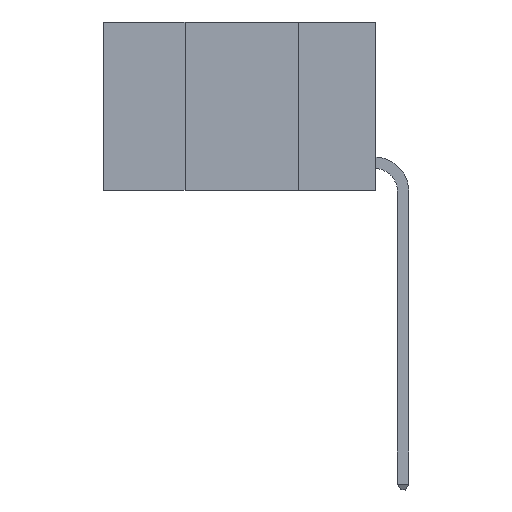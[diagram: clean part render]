
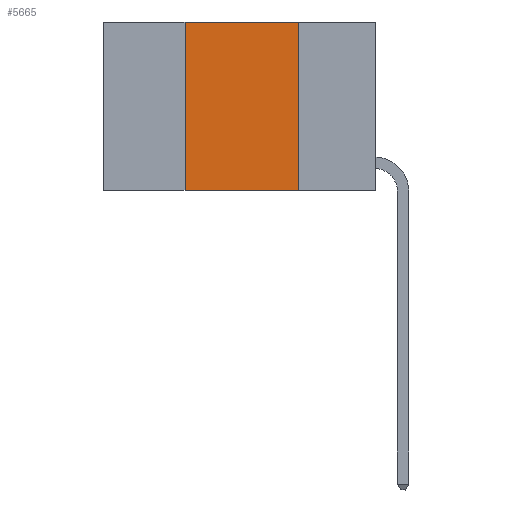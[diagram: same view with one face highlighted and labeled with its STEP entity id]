
A CAD part, left-side view. The second image highlights one B-rep face of the part: STEP entity #5665.
In plain terms, the highlighted planar face has unit normal (-1, 0, 0).
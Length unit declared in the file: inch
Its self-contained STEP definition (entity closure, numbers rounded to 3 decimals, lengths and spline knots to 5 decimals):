
#25 = LINE ( 'NONE', #11884, #8139 ) ;
#87 = EDGE_LOOP ( 'NONE', ( #11392, #12011, #11964, #6378 ) ) ;
#191 = LINE ( 'NONE', #9231, #8312 ) ;
#249 = VERTEX_POINT ( 'NONE', #7407 ) ;
#289 = LINE ( 'NONE', #11045, #2792 ) ;
#446 = PLANE ( 'NONE',  #7114 ) ;
#2586 = CARTESIAN_POINT ( 'NONE',  ( 0., 0.6, 0. ) ) ;
#2687 = VERTEX_POINT ( 'NONE', #5014 ) ;
#2792 = VECTOR ( 'NONE', #5935, 39.37008 ) ;
#3687 = DIRECTION ( 'NONE',  ( 0., 0., -1. ) ) ;
#5011 = VERTEX_POINT ( 'NONE', #9884 ) ;
#5014 = CARTESIAN_POINT ( 'NONE',  ( 0., 0.42, -0.37 ) ) ;
#5665 = ADVANCED_FACE ( 'NONE', ( #7409 ), #446, .F. ) ;
#5935 = DIRECTION ( 'NONE',  ( 0., -1., 0. ) ) ;
#6378 = ORIENTED_EDGE ( 'NONE', *, *, #9477, .T. ) ;
#7114 = AXIS2_PLACEMENT_3D ( 'NONE', #2586, #9945, #3687 ) ;
#7407 = CARTESIAN_POINT ( 'NONE',  ( 0., 0.42, 0. ) ) ;
#7409 = FACE_OUTER_BOUND ( 'NONE', #87, .T. ) ;
#7793 = DIRECTION ( 'NONE',  ( 0., 0., -1. ) ) ;
#7870 = VERTEX_POINT ( 'NONE', #9917 ) ;
#8139 = VECTOR ( 'NONE', #7793, 39.37008 ) ;
#8264 = DIRECTION ( 'NONE',  ( 0., -1., 0. ) ) ;
#8312 = VECTOR ( 'NONE', #13184, 39.37008 ) ;
#9140 = EDGE_CURVE ( 'NONE', #7870, #5011, #25, .T. ) ;
#9231 = CARTESIAN_POINT ( 'NONE',  ( 0., 0.42, 0. ) ) ;
#9272 = CARTESIAN_POINT ( 'NONE',  ( 0., 0.6, -0.37 ) ) ;
#9417 = EDGE_CURVE ( 'NONE', #2687, #249, #191, .T. ) ;
#9477 = EDGE_CURVE ( 'NONE', #2687, #5011, #13289, .T. ) ;
#9884 = CARTESIAN_POINT ( 'NONE',  ( 0., 0.17, -0.37 ) ) ;
#9917 = CARTESIAN_POINT ( 'NONE',  ( 0., 0.17, 0. ) ) ;
#9945 = DIRECTION ( 'NONE',  ( 1., 0., 0. ) ) ;
#10992 = VECTOR ( 'NONE', #8264, 39.37008 ) ;
#11045 = CARTESIAN_POINT ( 'NONE',  ( 0., 0.6, 0. ) ) ;
#11392 = ORIENTED_EDGE ( 'NONE', *, *, #9140, .F. ) ;
#11832 = EDGE_CURVE ( 'NONE', #249, #7870, #289, .T. ) ;
#11884 = CARTESIAN_POINT ( 'NONE',  ( 0., 0.17, 0. ) ) ;
#11964 = ORIENTED_EDGE ( 'NONE', *, *, #9417, .F. ) ;
#12011 = ORIENTED_EDGE ( 'NONE', *, *, #11832, .F. ) ;
#13184 = DIRECTION ( 'NONE',  ( 0., 0., 1. ) ) ;
#13289 = LINE ( 'NONE', #9272, #10992 ) ;
